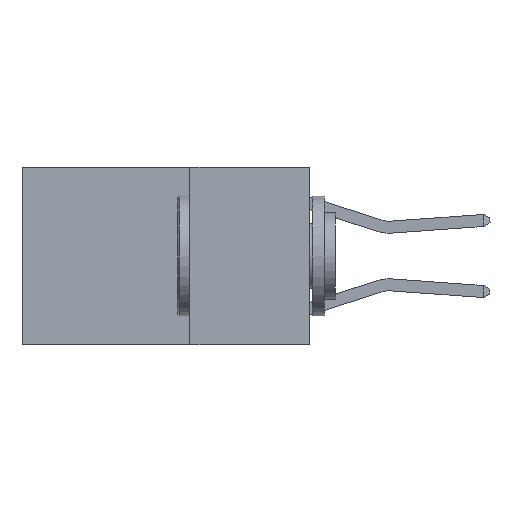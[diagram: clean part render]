
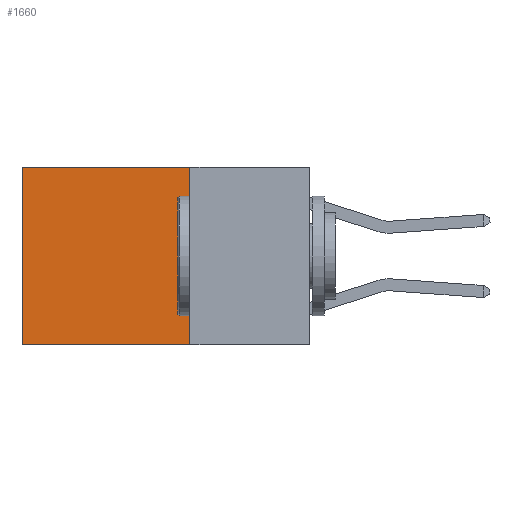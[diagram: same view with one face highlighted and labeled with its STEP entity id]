
A CAD part, left-side view. The second image highlights one B-rep face of the part: STEP entity #1660.
In plain terms, the highlighted planar face has unit normal (-1, 0, 0).
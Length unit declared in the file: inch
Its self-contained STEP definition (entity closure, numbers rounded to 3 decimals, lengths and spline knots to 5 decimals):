
#702 = CARTESIAN_POINT ( 'NONE',  ( 0.2625, 0.6, 0. ) ) ;
#1141 = CARTESIAN_POINT ( 'NONE',  ( 0.2625, 0.25, 0. ) ) ;
#1286 = CARTESIAN_POINT ( 'NONE',  ( 0.2625, 0.25, 0. ) ) ;
#1409 = CARTESIAN_POINT ( 'NONE',  ( 0.2625, 0.25, 0. ) ) ;
#1660 = ADVANCED_FACE ( 'NONE', ( #3952 ), #2580, .F. ) ;
#1682 = CARTESIAN_POINT ( 'NONE',  ( 0.2625, 0.25, 0. ) ) ;
#1717 = VECTOR ( 'NONE', #7212, 39.37008 ) ;
#1838 = LINE ( 'NONE', #702, #5399 ) ;
#1914 = DIRECTION ( 'NONE',  ( 0., 0., -1. ) ) ;
#2047 = LINE ( 'NONE', #8579, #1717 ) ;
#2530 = CARTESIAN_POINT ( 'NONE',  ( 0.2625, 0.25, -0.37 ) ) ;
#2580 = PLANE ( 'NONE',  #4481 ) ;
#2643 = VERTEX_POINT ( 'NONE', #8098 ) ;
#2942 = CARTESIAN_POINT ( 'NONE',  ( 0.2625, 0.6, -0.37 ) ) ;
#3177 = LINE ( 'NONE', #1286, #7322 ) ;
#3464 = EDGE_CURVE ( 'NONE', #4206, #2643, #3177, .T. ) ;
#3474 = EDGE_CURVE ( 'NONE', #4206, #5456, #4065, .T. ) ;
#3952 = FACE_OUTER_BOUND ( 'NONE', #6575, .T. ) ;
#4065 = LINE ( 'NONE', #1409, #4514 ) ;
#4166 = VERTEX_POINT ( 'NONE', #2942 ) ;
#4206 = VERTEX_POINT ( 'NONE', #1682 ) ;
#4358 = ORIENTED_EDGE ( 'NONE', *, *, #3464, .T. ) ;
#4481 = AXIS2_PLACEMENT_3D ( 'NONE', #1141, #6691, #1914 ) ;
#4514 = VECTOR ( 'NONE', #4825, 39.37008 ) ;
#4689 = DIRECTION ( 'NONE',  ( 0., 1., 0. ) ) ;
#4825 = DIRECTION ( 'NONE',  ( 0., 0., -1. ) ) ;
#4932 = EDGE_CURVE ( 'NONE', #2643, #4166, #1838, .T. ) ;
#5399 = VECTOR ( 'NONE', #8998, 39.37008 ) ;
#5456 = VERTEX_POINT ( 'NONE', #2530 ) ;
#6107 = ORIENTED_EDGE ( 'NONE', *, *, #4932, .T. ) ;
#6575 = EDGE_LOOP ( 'NONE', ( #6107, #7749, #8455, #4358 ) ) ;
#6691 = DIRECTION ( 'NONE',  ( 1., 0., 0. ) ) ;
#6865 = EDGE_CURVE ( 'NONE', #5456, #4166, #2047, .T. ) ;
#7212 = DIRECTION ( 'NONE',  ( 0., 1., 0. ) ) ;
#7322 = VECTOR ( 'NONE', #4689, 39.37008 ) ;
#7749 = ORIENTED_EDGE ( 'NONE', *, *, #6865, .F. ) ;
#8098 = CARTESIAN_POINT ( 'NONE',  ( 0.2625, 0.6, 0. ) ) ;
#8455 = ORIENTED_EDGE ( 'NONE', *, *, #3474, .F. ) ;
#8579 = CARTESIAN_POINT ( 'NONE',  ( 0.2625, 0.25, -0.37 ) ) ;
#8998 = DIRECTION ( 'NONE',  ( 0., 0., -1. ) ) ;
